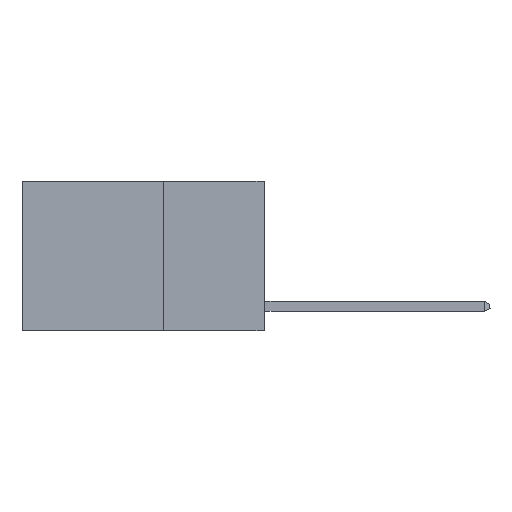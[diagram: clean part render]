
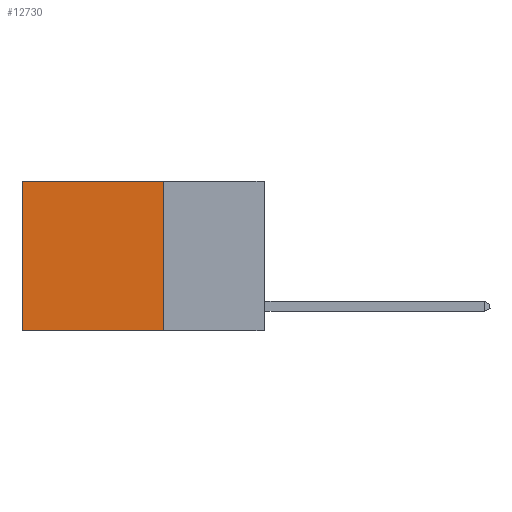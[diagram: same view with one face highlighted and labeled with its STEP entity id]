
A CAD part, left-side view. The second image highlights one B-rep face of the part: STEP entity #12730.
In plain terms, the highlighted planar face has unit normal (-1, 0, 0).
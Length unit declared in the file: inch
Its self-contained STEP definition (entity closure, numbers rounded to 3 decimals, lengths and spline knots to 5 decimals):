
#26 = ORIENTED_EDGE ( 'NONE', *, *, #8203, .F. ) ;
#74 = DIRECTION ( 'NONE',  ( 0., 0., -1. ) ) ;
#136 = VERTEX_POINT ( 'NONE', #13222 ) ;
#294 = CARTESIAN_POINT ( 'NONE',  ( 0.2625, 0.25, 0. ) ) ;
#1907 = LINE ( 'NONE', #2180, #6272 ) ;
#2180 = CARTESIAN_POINT ( 'NONE',  ( 0.2625, 0.25, 0. ) ) ;
#2201 = CARTESIAN_POINT ( 'NONE',  ( 0.2625, 0.25, 0. ) ) ;
#2475 = ORIENTED_EDGE ( 'NONE', *, *, #12700, .F. ) ;
#2817 = VERTEX_POINT ( 'NONE', #13372 ) ;
#3232 = CARTESIAN_POINT ( 'NONE',  ( 0.2625, 0.25, -0.37 ) ) ;
#3602 = VECTOR ( 'NONE', #10735, 39.37008 ) ;
#4027 = AXIS2_PLACEMENT_3D ( 'NONE', #294, #12138, #5708 ) ;
#4449 = PLANE ( 'NONE',  #4027 ) ;
#4543 = VERTEX_POINT ( 'NONE', #7841 ) ;
#5708 = DIRECTION ( 'NONE',  ( 0., 0., -1. ) ) ;
#5876 = ORIENTED_EDGE ( 'NONE', *, *, #9133, .T. ) ;
#6272 = VECTOR ( 'NONE', #74, 39.37008 ) ;
#6841 = CARTESIAN_POINT ( 'NONE',  ( 0.2625, 0.6, 0. ) ) ;
#7613 = LINE ( 'NONE', #2201, #7786 ) ;
#7786 = VECTOR ( 'NONE', #12932, 39.37008 ) ;
#7841 = CARTESIAN_POINT ( 'NONE',  ( 0.2625, 0.6, 0. ) ) ;
#8203 = EDGE_CURVE ( 'NONE', #136, #8771, #12846, .T. ) ;
#8771 = VERTEX_POINT ( 'NONE', #10788 ) ;
#9133 = EDGE_CURVE ( 'NONE', #4543, #8771, #10884, .T. ) ;
#10133 = DIRECTION ( 'NONE',  ( 0., 0., -1. ) ) ;
#10735 = DIRECTION ( 'NONE',  ( 0., 1., 0. ) ) ;
#10788 = CARTESIAN_POINT ( 'NONE',  ( 0.2625, 0.6, -0.37 ) ) ;
#10818 = FACE_OUTER_BOUND ( 'NONE', #11844, .T. ) ;
#10884 = LINE ( 'NONE', #6841, #13255 ) ;
#11844 = EDGE_LOOP ( 'NONE', ( #5876, #26, #2475, #11973 ) ) ;
#11973 = ORIENTED_EDGE ( 'NONE', *, *, #12292, .T. ) ;
#12138 = DIRECTION ( 'NONE',  ( 1., 0., 0. ) ) ;
#12292 = EDGE_CURVE ( 'NONE', #2817, #4543, #7613, .T. ) ;
#12700 = EDGE_CURVE ( 'NONE', #2817, #136, #1907, .T. ) ;
#12730 = ADVANCED_FACE ( 'NONE', ( #10818 ), #4449, .F. ) ;
#12846 = LINE ( 'NONE', #3232, #3602 ) ;
#12932 = DIRECTION ( 'NONE',  ( 0., 1., 0. ) ) ;
#13222 = CARTESIAN_POINT ( 'NONE',  ( 0.2625, 0.25, -0.37 ) ) ;
#13255 = VECTOR ( 'NONE', #10133, 39.37008 ) ;
#13372 = CARTESIAN_POINT ( 'NONE',  ( 0.2625, 0.25, 0. ) ) ;
